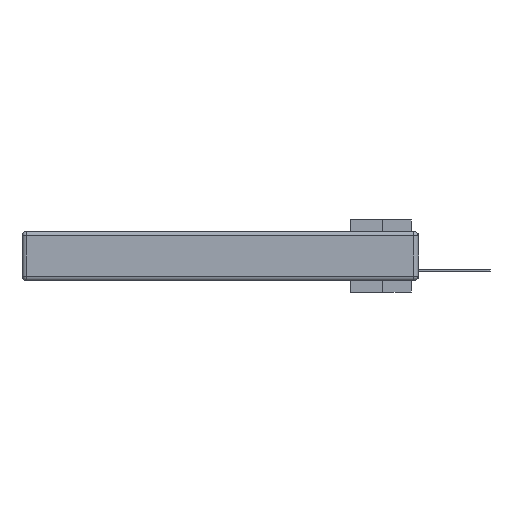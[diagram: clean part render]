
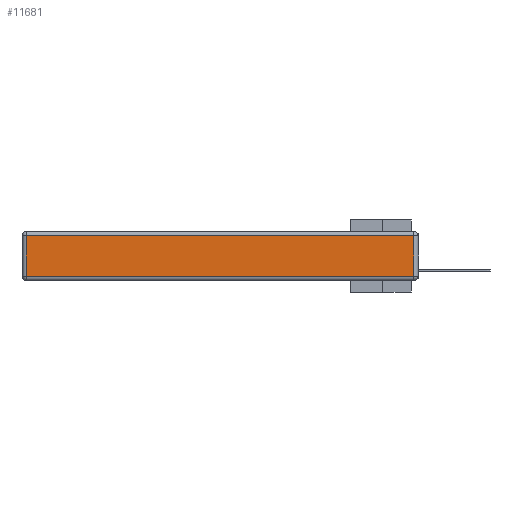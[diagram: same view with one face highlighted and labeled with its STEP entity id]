
A CAD part, left-side view. The second image highlights one B-rep face of the part: STEP entity #11681.
In plain terms, the highlighted planar face has unit normal (-1, 0, 0).
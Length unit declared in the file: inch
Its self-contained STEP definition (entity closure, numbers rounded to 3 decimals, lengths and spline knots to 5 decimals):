
#1789 = CARTESIAN_POINT ( 'NONE',  ( 0., 0., -0.343 ) ) ;
#1934 = LINE ( 'NONE', #9256, #20934 ) ;
#2983 = LINE ( 'NONE', #7920, #21922 ) ;
#3286 = EDGE_CURVE ( 'NONE', #18713, #8773, #1934, .T. ) ;
#3750 = CARTESIAN_POINT ( 'NONE',  ( 0., 0.03, -0.343 ) ) ;
#5496 = EDGE_LOOP ( 'NONE', ( #5659, #16739, #14950, #20802 ) ) ;
#5659 = ORIENTED_EDGE ( 'NONE', *, *, #8613, .T. ) ;
#7527 = VECTOR ( 'NONE', #8369, 39.37008 ) ;
#7603 = LINE ( 'NONE', #19680, #15368 ) ;
#7920 = CARTESIAN_POINT ( 'NONE',  ( 0., 2.72, -0.343 ) ) ;
#8369 = DIRECTION ( 'NONE',  ( 0., 0., 1. ) ) ;
#8613 = EDGE_CURVE ( 'NONE', #11614, #20478, #7603, .T. ) ;
#8773 = VERTEX_POINT ( 'NONE', #22706 ) ;
#8830 = LINE ( 'NONE', #3750, #7527 ) ;
#9256 = CARTESIAN_POINT ( 'NONE',  ( 0., 2.75, -0.03 ) ) ;
#11614 = VERTEX_POINT ( 'NONE', #28172 ) ;
#11643 = DIRECTION ( 'NONE',  ( 0., 0., 1. ) ) ;
#11681 = ADVANCED_FACE ( 'NONE', ( #23748 ), #28802, .T. ) ;
#12685 = DIRECTION ( 'NONE',  ( 0., -1., 0. ) ) ;
#13984 = EDGE_CURVE ( 'NONE', #20478, #18713, #8830, .T. ) ;
#14950 = ORIENTED_EDGE ( 'NONE', *, *, #3286, .T. ) ;
#15011 = AXIS2_PLACEMENT_3D ( 'NONE', #1789, #19288, #11643 ) ;
#15175 = CARTESIAN_POINT ( 'NONE',  ( 0., 0.03, -0.03 ) ) ;
#15368 = VECTOR ( 'NONE', #12685, 39.37008 ) ;
#16739 = ORIENTED_EDGE ( 'NONE', *, *, #13984, .T. ) ;
#17607 = DIRECTION ( 'NONE',  ( 0., 0., -1. ) ) ;
#18713 = VERTEX_POINT ( 'NONE', #15175 ) ;
#18957 = DIRECTION ( 'NONE',  ( 0., 1., 0. ) ) ;
#19288 = DIRECTION ( 'NONE',  ( -1., 0., 0. ) ) ;
#19680 = CARTESIAN_POINT ( 'NONE',  ( 0., 0., -0.313 ) ) ;
#20478 = VERTEX_POINT ( 'NONE', #27998 ) ;
#20802 = ORIENTED_EDGE ( 'NONE', *, *, #27230, .T. ) ;
#20934 = VECTOR ( 'NONE', #18957, 39.37008 ) ;
#21922 = VECTOR ( 'NONE', #17607, 39.37008 ) ;
#22706 = CARTESIAN_POINT ( 'NONE',  ( 0., 2.72, -0.03 ) ) ;
#23748 = FACE_OUTER_BOUND ( 'NONE', #5496, .T. ) ;
#27230 = EDGE_CURVE ( 'NONE', #8773, #11614, #2983, .T. ) ;
#27998 = CARTESIAN_POINT ( 'NONE',  ( 0., 0.03, -0.313 ) ) ;
#28172 = CARTESIAN_POINT ( 'NONE',  ( 0., 2.72, -0.313 ) ) ;
#28802 = PLANE ( 'NONE',  #15011 ) ;
